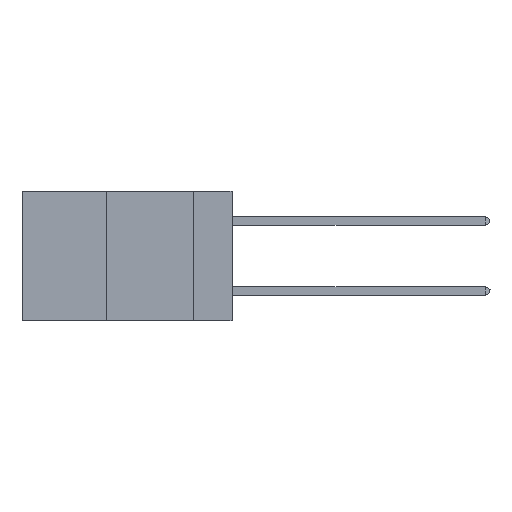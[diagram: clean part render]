
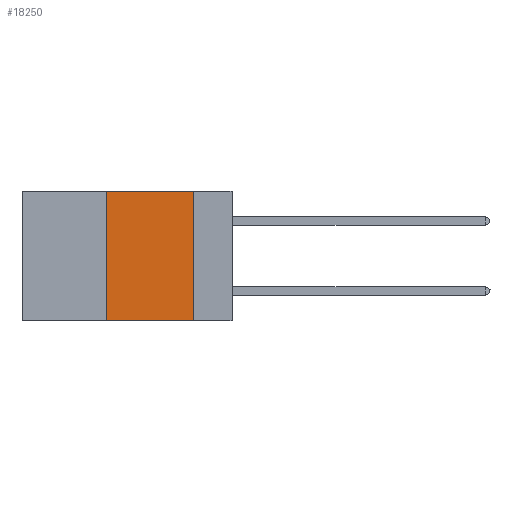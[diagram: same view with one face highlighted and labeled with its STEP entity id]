
A CAD part, left-side view. The second image highlights one B-rep face of the part: STEP entity #18250.
In plain terms, the highlighted planar face has unit normal (-1, 0, 0).
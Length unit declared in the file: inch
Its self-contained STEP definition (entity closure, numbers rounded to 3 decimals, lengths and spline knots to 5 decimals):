
#629 = ORIENTED_EDGE ( 'NONE', *, *, #31468, .F. ) ;
#910 = PLANE ( 'NONE',  #1691 ) ;
#1454 = DIRECTION ( 'NONE',  ( 0., 0., 1. ) ) ;
#1630 = VECTOR ( 'NONE', #1454, 39.37008 ) ;
#1691 = AXIS2_PLACEMENT_3D ( 'NONE', #32220, #12762, #12568 ) ;
#1913 = DIRECTION ( 'NONE',  ( 0., -1., 0. ) ) ;
#2421 = LINE ( 'NONE', #5616, #34068 ) ;
#3257 = VERTEX_POINT ( 'NONE', #11142 ) ;
#4831 = LINE ( 'NONE', #33514, #1630 ) ;
#4836 = CARTESIAN_POINT ( 'NONE',  ( 0., 0.11, 0. ) ) ;
#5616 = CARTESIAN_POINT ( 'NONE',  ( 0., 0.11, 0. ) ) ;
#9072 = ORIENTED_EDGE ( 'NONE', *, *, #36013, .F. ) ;
#10334 = VECTOR ( 'NONE', #1913, 39.37008 ) ;
#11142 = CARTESIAN_POINT ( 'NONE',  ( 0., 0.36, -0.37 ) ) ;
#12568 = DIRECTION ( 'NONE',  ( 0., 0., -1. ) ) ;
#12762 = DIRECTION ( 'NONE',  ( 1., 0., 0. ) ) ;
#13211 = LINE ( 'NONE', #13587, #10334 ) ;
#13587 = CARTESIAN_POINT ( 'NONE',  ( 0., 0.6, -0.37 ) ) ;
#14924 = CARTESIAN_POINT ( 'NONE',  ( 0., 0.36, 0. ) ) ;
#15911 = CARTESIAN_POINT ( 'NONE',  ( 0., 0.11, -0.37 ) ) ;
#16208 = VECTOR ( 'NONE', #16481, 39.37008 ) ;
#16260 = ORIENTED_EDGE ( 'NONE', *, *, #24585, .T. ) ;
#16481 = DIRECTION ( 'NONE',  ( 0., -1., 0. ) ) ;
#18250 = ADVANCED_FACE ( 'NONE', ( #26925 ), #910, .F. ) ;
#23350 = EDGE_LOOP ( 'NONE', ( #629, #9072, #31848, #16260 ) ) ;
#24585 = EDGE_CURVE ( 'NONE', #3257, #33540, #13211, .T. ) ;
#25170 = LINE ( 'NONE', #28004, #16208 ) ;
#26925 = FACE_OUTER_BOUND ( 'NONE', #23350, .T. ) ;
#28004 = CARTESIAN_POINT ( 'NONE',  ( 0., 0.6, 0. ) ) ;
#31468 = EDGE_CURVE ( 'NONE', #35542, #33540, #2421, .T. ) ;
#31848 = ORIENTED_EDGE ( 'NONE', *, *, #33159, .F. ) ;
#31956 = VERTEX_POINT ( 'NONE', #14924 ) ;
#32220 = CARTESIAN_POINT ( 'NONE',  ( 0., 0.6, 0. ) ) ;
#33159 = EDGE_CURVE ( 'NONE', #3257, #31956, #4831, .T. ) ;
#33514 = CARTESIAN_POINT ( 'NONE',  ( 0., 0.36, 0. ) ) ;
#33540 = VERTEX_POINT ( 'NONE', #15911 ) ;
#33930 = DIRECTION ( 'NONE',  ( 0., 0., -1. ) ) ;
#34068 = VECTOR ( 'NONE', #33930, 39.37008 ) ;
#35542 = VERTEX_POINT ( 'NONE', #4836 ) ;
#36013 = EDGE_CURVE ( 'NONE', #31956, #35542, #25170, .T. ) ;
